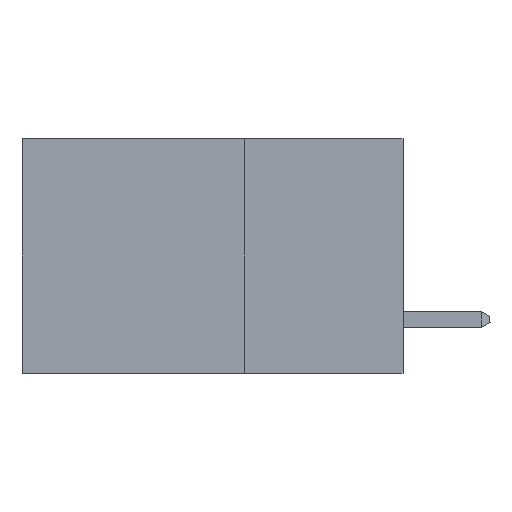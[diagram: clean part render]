
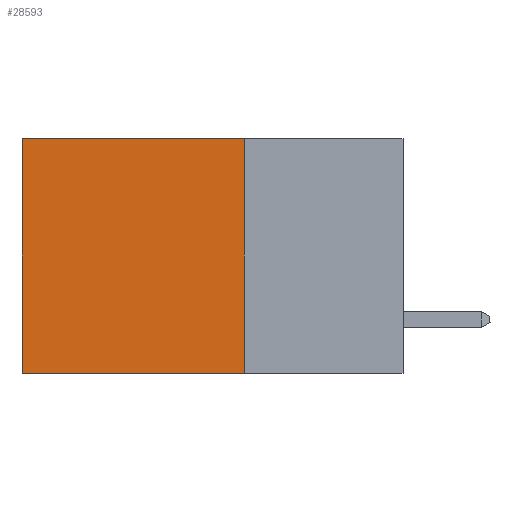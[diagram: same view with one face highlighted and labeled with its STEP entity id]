
A CAD part, left-side view. The second image highlights one B-rep face of the part: STEP entity #28593.
In plain terms, the highlighted planar face has unit normal (-1, 0, 0).
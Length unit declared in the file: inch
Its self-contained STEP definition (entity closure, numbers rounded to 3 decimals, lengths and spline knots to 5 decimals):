
#1114 = VERTEX_POINT ( 'NONE', #11020 ) ;
#3694 = EDGE_LOOP ( 'NONE', ( #35836, #26603, #7345, #4417 ) ) ;
#4417 = ORIENTED_EDGE ( 'NONE', *, *, #4730, .T. ) ;
#4730 = EDGE_CURVE ( 'NONE', #23570, #39483, #5648, .T. ) ;
#5091 = CARTESIAN_POINT ( 'NONE',  ( 0.2875, 0.25, -0.37 ) ) ;
#5648 = LINE ( 'NONE', #13154, #37218 ) ;
#7181 = DIRECTION ( 'NONE',  ( 0., 0., -1. ) ) ;
#7345 = ORIENTED_EDGE ( 'NONE', *, *, #17824, .F. ) ;
#8115 = DIRECTION ( 'NONE',  ( 0., 0., -1. ) ) ;
#8325 = VERTEX_POINT ( 'NONE', #5091 ) ;
#8468 = EDGE_CURVE ( 'NONE', #8325, #1114, #36443, .T. ) ;
#11020 = CARTESIAN_POINT ( 'NONE',  ( 0.2875, 0.6, -0.37 ) ) ;
#11082 = VECTOR ( 'NONE', #8115, 39.37008 ) ;
#11216 = AXIS2_PLACEMENT_3D ( 'NONE', #18670, #24636, #24759 ) ;
#11954 = DIRECTION ( 'NONE',  ( 0., 1., 0. ) ) ;
#13154 = CARTESIAN_POINT ( 'NONE',  ( 0.2875, 0.25, 0. ) ) ;
#17506 = CARTESIAN_POINT ( 'NONE',  ( 0.2875, 0.25, 0. ) ) ;
#17824 = EDGE_CURVE ( 'NONE', #23570, #8325, #20422, .T. ) ;
#18670 = CARTESIAN_POINT ( 'NONE',  ( 0.2875, 0.25, 0. ) ) ;
#19390 = VECTOR ( 'NONE', #11954, 39.37008 ) ;
#19433 = DIRECTION ( 'NONE',  ( 0., 1., 0. ) ) ;
#20422 = LINE ( 'NONE', #31549, #21376 ) ;
#21376 = VECTOR ( 'NONE', #7181, 39.37008 ) ;
#21730 = PLANE ( 'NONE',  #11216 ) ;
#23570 = VERTEX_POINT ( 'NONE', #17506 ) ;
#24636 = DIRECTION ( 'NONE',  ( 1., 0., 0. ) ) ;
#24759 = DIRECTION ( 'NONE',  ( 0., 0., -1. ) ) ;
#26603 = ORIENTED_EDGE ( 'NONE', *, *, #8468, .F. ) ;
#27249 = CARTESIAN_POINT ( 'NONE',  ( 0.2875, 0.25, -0.37 ) ) ;
#28593 = ADVANCED_FACE ( 'NONE', ( #39114 ), #21730, .F. ) ;
#29538 = CARTESIAN_POINT ( 'NONE',  ( 0.2875, 0.6, 0. ) ) ;
#31549 = CARTESIAN_POINT ( 'NONE',  ( 0.2875, 0.25, 0. ) ) ;
#33024 = EDGE_CURVE ( 'NONE', #39483, #1114, #35487, .T. ) ;
#35487 = LINE ( 'NONE', #29538, #11082 ) ;
#35836 = ORIENTED_EDGE ( 'NONE', *, *, #33024, .T. ) ;
#36443 = LINE ( 'NONE', #27249, #19390 ) ;
#37218 = VECTOR ( 'NONE', #19433, 39.37008 ) ;
#38182 = CARTESIAN_POINT ( 'NONE',  ( 0.2875, 0.6, 0. ) ) ;
#39114 = FACE_OUTER_BOUND ( 'NONE', #3694, .T. ) ;
#39483 = VERTEX_POINT ( 'NONE', #38182 ) ;
